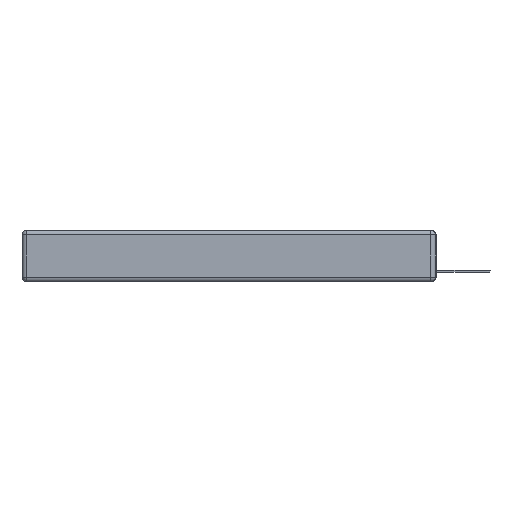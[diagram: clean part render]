
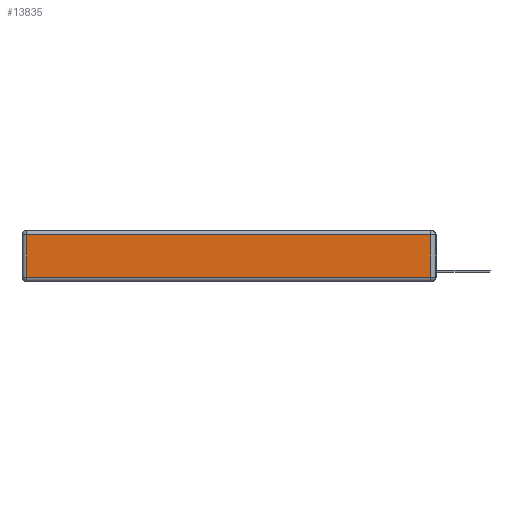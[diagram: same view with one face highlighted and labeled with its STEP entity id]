
A CAD part, left-side view. The second image highlights one B-rep face of the part: STEP entity #13835.
In plain terms, the highlighted planar face has unit normal (-1, 0, 0).
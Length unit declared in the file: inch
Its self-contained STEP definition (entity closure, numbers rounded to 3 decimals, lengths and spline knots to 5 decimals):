
#149 = ORIENTED_EDGE ( 'NONE', *, *, #15947, .T. ) ;
#1337 = EDGE_CURVE ( 'NONE', #14401, #21408, #13020, .T. ) ;
#1358 = DIRECTION ( 'NONE',  ( 0., 0., -1. ) ) ;
#2379 = LINE ( 'NONE', #15108, #20263 ) ;
#2798 = CARTESIAN_POINT ( 'NONE',  ( 0., 0.03, -0.343 ) ) ;
#3355 = DIRECTION ( 'NONE',  ( 0., 0., 1. ) ) ;
#4504 = EDGE_LOOP ( 'NONE', ( #16511, #149, #15660, #16292 ) ) ;
#4533 = VECTOR ( 'NONE', #14521, 39.37008 ) ;
#6092 = LINE ( 'NONE', #8599, #4533 ) ;
#6411 = EDGE_CURVE ( 'NONE', #23652, #14401, #2379, .T. ) ;
#7674 = CARTESIAN_POINT ( 'NONE',  ( 0., 0.03, -0.03 ) ) ;
#8294 = VECTOR ( 'NONE', #16830, 39.37008 ) ;
#8366 = DIRECTION ( 'NONE',  ( 0., -1., 0. ) ) ;
#8599 = CARTESIAN_POINT ( 'NONE',  ( 0., 2.75, -0.03 ) ) ;
#10540 = FACE_OUTER_BOUND ( 'NONE', #4504, .T. ) ;
#11623 = CARTESIAN_POINT ( 'NONE',  ( 0., 0., -0.343 ) ) ;
#11838 = CARTESIAN_POINT ( 'NONE',  ( 0., 0.03, -0.313 ) ) ;
#12632 = AXIS2_PLACEMENT_3D ( 'NONE', #11623, #25236, #3355 ) ;
#13020 = LINE ( 'NONE', #24752, #17980 ) ;
#13835 = ADVANCED_FACE ( 'NONE', ( #10540 ), #17497, .T. ) ;
#14401 = VERTEX_POINT ( 'NONE', #15675 ) ;
#14521 = DIRECTION ( 'NONE',  ( 0., 1., 0. ) ) ;
#14817 = CARTESIAN_POINT ( 'NONE',  ( 0., 2.72, -0.03 ) ) ;
#15108 = CARTESIAN_POINT ( 'NONE',  ( 0., 2.72, -0.343 ) ) ;
#15368 = LINE ( 'NONE', #2798, #8294 ) ;
#15660 = ORIENTED_EDGE ( 'NONE', *, *, #17126, .T. ) ;
#15675 = CARTESIAN_POINT ( 'NONE',  ( 0., 2.72, -0.313 ) ) ;
#15947 = EDGE_CURVE ( 'NONE', #21408, #18901, #15368, .T. ) ;
#16292 = ORIENTED_EDGE ( 'NONE', *, *, #6411, .T. ) ;
#16511 = ORIENTED_EDGE ( 'NONE', *, *, #1337, .T. ) ;
#16830 = DIRECTION ( 'NONE',  ( 0., 0., 1. ) ) ;
#17126 = EDGE_CURVE ( 'NONE', #18901, #23652, #6092, .T. ) ;
#17497 = PLANE ( 'NONE',  #12632 ) ;
#17980 = VECTOR ( 'NONE', #8366, 39.37008 ) ;
#18901 = VERTEX_POINT ( 'NONE', #7674 ) ;
#20263 = VECTOR ( 'NONE', #1358, 39.37008 ) ;
#21408 = VERTEX_POINT ( 'NONE', #11838 ) ;
#23652 = VERTEX_POINT ( 'NONE', #14817 ) ;
#24752 = CARTESIAN_POINT ( 'NONE',  ( 0., 0., -0.313 ) ) ;
#25236 = DIRECTION ( 'NONE',  ( -1., 0., 0. ) ) ;
